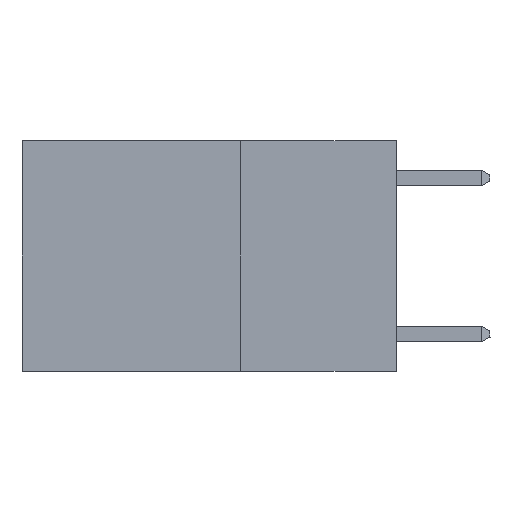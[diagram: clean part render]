
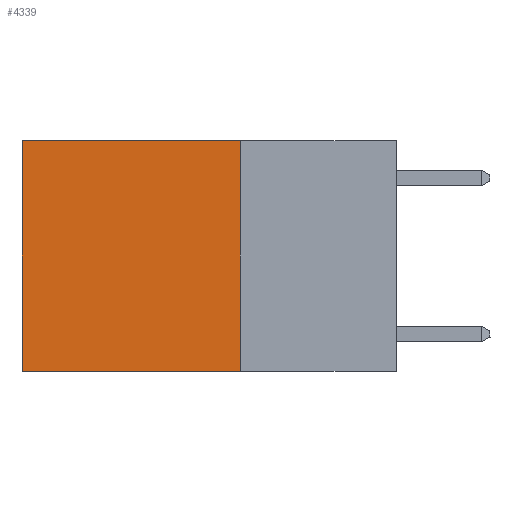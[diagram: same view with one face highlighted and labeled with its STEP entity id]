
A CAD part, left-side view. The second image highlights one B-rep face of the part: STEP entity #4339.
In plain terms, the highlighted planar face has unit normal (-1, 0, 0).
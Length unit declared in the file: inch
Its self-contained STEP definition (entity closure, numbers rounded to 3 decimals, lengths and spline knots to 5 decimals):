
#558 = CARTESIAN_POINT ( 'NONE',  ( 0.2625, 0.25, 0. ) ) ;
#2461 = CARTESIAN_POINT ( 'NONE',  ( 0.2625, 0.25, 0. ) ) ;
#2869 = VERTEX_POINT ( 'NONE', #10294 ) ;
#3219 = PLANE ( 'NONE',  #9075 ) ;
#3519 = EDGE_LOOP ( 'NONE', ( #3739, #3784, #3832, #3843 ) ) ;
#3566 = VECTOR ( 'NONE', #12013, 39.37008 ) ;
#3739 = ORIENTED_EDGE ( 'NONE', *, *, #11046, .T. ) ;
#3784 = ORIENTED_EDGE ( 'NONE', *, *, #6779, .F. ) ;
#3832 = ORIENTED_EDGE ( 'NONE', *, *, #4695, .F. ) ;
#3843 = ORIENTED_EDGE ( 'NONE', *, *, #7097, .T. ) ;
#4267 = DIRECTION ( 'NONE',  ( 0., 0., -1. ) ) ;
#4339 = ADVANCED_FACE ( 'NONE', ( #10503 ), #3219, .F. ) ;
#4438 = CARTESIAN_POINT ( 'NONE',  ( 0.2625, 0.25, -0.37 ) ) ;
#4646 = VECTOR ( 'NONE', #7298, 39.37008 ) ;
#4695 = EDGE_CURVE ( 'NONE', #12447, #5124, #9081, .T. ) ;
#4980 = LINE ( 'NONE', #5222, #4646 ) ;
#5124 = VERTEX_POINT ( 'NONE', #4438 ) ;
#5222 = CARTESIAN_POINT ( 'NONE',  ( 0.2625, 0.25, -0.37 ) ) ;
#5761 = CARTESIAN_POINT ( 'NONE',  ( 0.2625, 0.25, 0. ) ) ;
#6343 = CARTESIAN_POINT ( 'NONE',  ( 0.2625, 0.25, 0. ) ) ;
#6779 = EDGE_CURVE ( 'NONE', #5124, #10987, #4980, .T. ) ;
#7097 = EDGE_CURVE ( 'NONE', #12447, #2869, #8695, .T. ) ;
#7298 = DIRECTION ( 'NONE',  ( 0., 1., 0. ) ) ;
#8372 = VECTOR ( 'NONE', #12903, 39.37008 ) ;
#8695 = LINE ( 'NONE', #5761, #8372 ) ;
#8714 = CARTESIAN_POINT ( 'NONE',  ( 0.2625, 0.6, -0.37 ) ) ;
#9074 = VECTOR ( 'NONE', #12867, 39.37008 ) ;
#9075 = AXIS2_PLACEMENT_3D ( 'NONE', #6343, #10435, #4267 ) ;
#9081 = LINE ( 'NONE', #558, #3566 ) ;
#9390 = LINE ( 'NONE', #11816, #9074 ) ;
#10294 = CARTESIAN_POINT ( 'NONE',  ( 0.2625, 0.6, 0. ) ) ;
#10435 = DIRECTION ( 'NONE',  ( 1., 0., 0. ) ) ;
#10503 = FACE_OUTER_BOUND ( 'NONE', #3519, .T. ) ;
#10987 = VERTEX_POINT ( 'NONE', #8714 ) ;
#11046 = EDGE_CURVE ( 'NONE', #2869, #10987, #9390, .T. ) ;
#11816 = CARTESIAN_POINT ( 'NONE',  ( 0.2625, 0.6, 0. ) ) ;
#12013 = DIRECTION ( 'NONE',  ( 0., 0., -1. ) ) ;
#12447 = VERTEX_POINT ( 'NONE', #2461 ) ;
#12867 = DIRECTION ( 'NONE',  ( 0., 0., -1. ) ) ;
#12903 = DIRECTION ( 'NONE',  ( 0., 1., 0. ) ) ;
